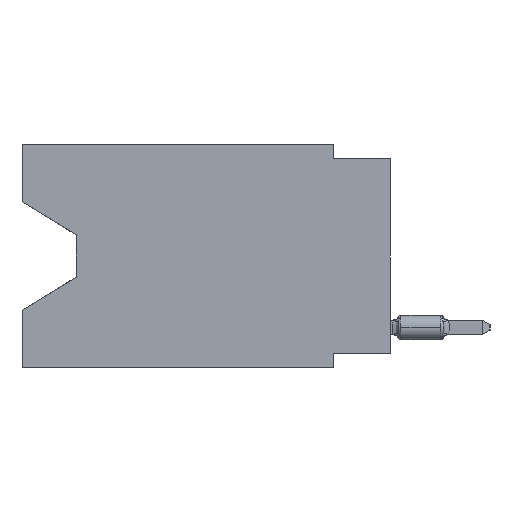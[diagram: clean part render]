
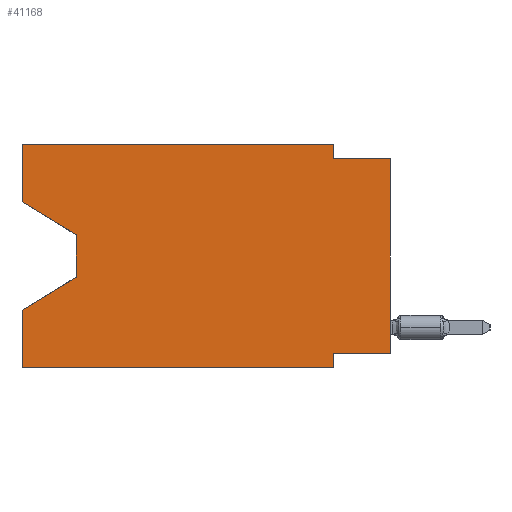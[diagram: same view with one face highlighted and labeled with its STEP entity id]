
A CAD part, left-side view. The second image highlights one B-rep face of the part: STEP entity #41168.
In plain terms, the highlighted planar face has unit normal (-1, 0, 0).
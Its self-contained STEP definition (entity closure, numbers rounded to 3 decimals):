
#561 = EDGE_CURVE ( 'NONE', #10498, #40357, #6008, .T. ) ;
#677 = DIRECTION ( 'NONE',  ( 0., -0.855, -0.519 ) ) ;
#1276 = CARTESIAN_POINT ( 'NONE',  ( 0., 0., 0. ) ) ;
#1778 = CARTESIAN_POINT ( 'NONE',  ( 0., 13.97, -4.013 ) ) ;
#1964 = CARTESIAN_POINT ( 'NONE',  ( 0., 0., -9.271 ) ) ;
#2694 = VERTEX_POINT ( 'NONE', #9017 ) ;
#3584 = VECTOR ( 'NONE', #27656, 1000. ) ;
#3711 = ORIENTED_EDGE ( 'NONE', *, *, #38095, .F. ) ;
#3873 = ORIENTED_EDGE ( 'NONE', *, *, #47036, .F. ) ;
#3886 = CARTESIAN_POINT ( 'NONE',  ( 0., 13.97, -5.893 ) ) ;
#4195 = LINE ( 'NONE', #28365, #49214 ) ;
#4669 = EDGE_CURVE ( 'NONE', #34271, #47103, #37674, .T. ) ;
#5193 = FACE_OUTER_BOUND ( 'NONE', #19505, .T. ) ;
#5781 = CARTESIAN_POINT ( 'NONE',  ( 0., 16.383, 0. ) ) ;
#6008 = LINE ( 'NONE', #1778, #26096 ) ;
#6830 = VECTOR ( 'NONE', #31070, 1000. ) ;
#7678 = VECTOR ( 'NONE', #21183, 1000. ) ;
#8118 = DIRECTION ( 'NONE',  ( 0., 0.855, -0.519 ) ) ;
#8648 = ORIENTED_EDGE ( 'NONE', *, *, #561, .T. ) ;
#9017 = CARTESIAN_POINT ( 'NONE',  ( 0., 16.383, -9.906 ) ) ;
#9403 = CARTESIAN_POINT ( 'NONE',  ( 0., 16.383, 0. ) ) ;
#10498 = VERTEX_POINT ( 'NONE', #44036 ) ;
#11215 = DIRECTION ( 'NONE',  ( 0., 0., -1. ) ) ;
#11441 = CARTESIAN_POINT ( 'NONE',  ( 0., 16.383, 0. ) ) ;
#11472 = CARTESIAN_POINT ( 'NONE',  ( 0., 2.54, 0. ) ) ;
#11843 = CARTESIAN_POINT ( 'NONE',  ( 0., 16.383, -7.36 ) ) ;
#12402 = CARTESIAN_POINT ( 'NONE',  ( 0., 2.54, -9.271 ) ) ;
#14045 = CARTESIAN_POINT ( 'NONE',  ( 0., 16.383, -9.906 ) ) ;
#14407 = ORIENTED_EDGE ( 'NONE', *, *, #51488, .F. ) ;
#16347 = ORIENTED_EDGE ( 'NONE', *, *, #43028, .T. ) ;
#16636 = ORIENTED_EDGE ( 'NONE', *, *, #39897, .T. ) ;
#16819 = DIRECTION ( 'NONE',  ( 0., 1., 0. ) ) ;
#17149 = VERTEX_POINT ( 'NONE', #5781 ) ;
#17970 = VERTEX_POINT ( 'NONE', #35921 ) ;
#18001 = CARTESIAN_POINT ( 'NONE',  ( 0., 0., -0.635 ) ) ;
#18196 = DIRECTION ( 'NONE',  ( 1., 0., 0. ) ) ;
#19505 = EDGE_LOOP ( 'NONE', ( #16636, #8648, #44319, #31109, #16347, #34948, #3711, #27749, #3873, #35640, #29774, #14407 ) ) ;
#20395 = DIRECTION ( 'NONE',  ( 0., 0., 1. ) ) ;
#20474 = VERTEX_POINT ( 'NONE', #37062 ) ;
#21049 = LINE ( 'NONE', #3886, #47993 ) ;
#21183 = DIRECTION ( 'NONE',  ( 0., -1., 0. ) ) ;
#21549 = EDGE_CURVE ( 'NONE', #26577, #20474, #44074, .T. ) ;
#22024 = LINE ( 'NONE', #14045, #49543 ) ;
#24725 = CARTESIAN_POINT ( 'NONE',  ( 0., 13.97, -5.893 ) ) ;
#25175 = CARTESIAN_POINT ( 'NONE',  ( 0., 0., -0.635 ) ) ;
#25344 = EDGE_CURVE ( 'NONE', #2694, #36267, #4195, .T. ) ;
#26096 = VECTOR ( 'NONE', #50118, 1000. ) ;
#26577 = VERTEX_POINT ( 'NONE', #12402 ) ;
#27268 = CARTESIAN_POINT ( 'NONE',  ( 0., 2.54, -0.635 ) ) ;
#27656 = DIRECTION ( 'NONE',  ( 0., 0., 1. ) ) ;
#27749 = ORIENTED_EDGE ( 'NONE', *, *, #4669, .T. ) ;
#28365 = CARTESIAN_POINT ( 'NONE',  ( 0., 16.383, 0. ) ) ;
#28625 = LINE ( 'NONE', #25175, #7678 ) ;
#29295 = LINE ( 'NONE', #45507, #32343 ) ;
#29618 = DIRECTION ( 'NONE',  ( 0., 0., -1. ) ) ;
#29774 = ORIENTED_EDGE ( 'NONE', *, *, #46326, .F. ) ;
#31070 = DIRECTION ( 'NONE',  ( 0., 0., -1. ) ) ;
#31109 = ORIENTED_EDGE ( 'NONE', *, *, #25344, .F. ) ;
#32343 = VECTOR ( 'NONE', #16819, 1000. ) ;
#34110 = LINE ( 'NONE', #9403, #47356 ) ;
#34271 = VERTEX_POINT ( 'NONE', #1964 ) ;
#34670 = CARTESIAN_POINT ( 'NONE',  ( 0., 16.383, 0. ) ) ;
#34948 = ORIENTED_EDGE ( 'NONE', *, *, #21549, .F. ) ;
#35640 = ORIENTED_EDGE ( 'NONE', *, *, #38329, .F. ) ;
#35921 = CARTESIAN_POINT ( 'NONE',  ( 0., 2.54, 0. ) ) ;
#36267 = VERTEX_POINT ( 'NONE', #11843 ) ;
#37062 = CARTESIAN_POINT ( 'NONE',  ( 0., 2.54, -9.906 ) ) ;
#37508 = CARTESIAN_POINT ( 'NONE',  ( 0., 16.383, -2.546 ) ) ;
#37674 = LINE ( 'NONE', #1276, #44317 ) ;
#38095 = EDGE_CURVE ( 'NONE', #34271, #26577, #29295, .T. ) ;
#38329 = EDGE_CURVE ( 'NONE', #17970, #52236, #47886, .T. ) ;
#39897 = EDGE_CURVE ( 'NONE', #43920, #10498, #44270, .T. ) ;
#40280 = CARTESIAN_POINT ( 'NONE',  ( 0., 16.383, -2.546 ) ) ;
#40357 = VERTEX_POINT ( 'NONE', #24725 ) ;
#41168 = ADVANCED_FACE ( 'NONE', ( #5193 ), #41849, .F. ) ;
#41822 = DIRECTION ( 'NONE',  ( 0., -1., 0. ) ) ;
#41849 = PLANE ( 'NONE',  #47034 ) ;
#43028 = EDGE_CURVE ( 'NONE', #2694, #20474, #22024, .T. ) ;
#43356 = LINE ( 'NONE', #11441, #3584 ) ;
#43920 = VERTEX_POINT ( 'NONE', #37508 ) ;
#44036 = CARTESIAN_POINT ( 'NONE',  ( 0., 13.97, -4.013 ) ) ;
#44074 = LINE ( 'NONE', #51516, #6830 ) ;
#44270 = LINE ( 'NONE', #40280, #48638 ) ;
#44317 = VECTOR ( 'NONE', #49880, 1000. ) ;
#44319 = ORIENTED_EDGE ( 'NONE', *, *, #52370, .T. ) ;
#45507 = CARTESIAN_POINT ( 'NONE',  ( 0., 0., -9.271 ) ) ;
#46326 = EDGE_CURVE ( 'NONE', #17149, #17970, #34110, .T. ) ;
#46473 = DIRECTION ( 'NONE',  ( 0., -1., 0. ) ) ;
#47034 = AXIS2_PLACEMENT_3D ( 'NONE', #34670, #18196, #29618 ) ;
#47036 = EDGE_CURVE ( 'NONE', #52236, #47103, #28625, .T. ) ;
#47103 = VERTEX_POINT ( 'NONE', #18001 ) ;
#47356 = VECTOR ( 'NONE', #41822, 1000. ) ;
#47886 = LINE ( 'NONE', #11472, #50203 ) ;
#47993 = VECTOR ( 'NONE', #8118, 1000. ) ;
#48638 = VECTOR ( 'NONE', #677, 1000. ) ;
#49214 = VECTOR ( 'NONE', #20395, 1000. ) ;
#49543 = VECTOR ( 'NONE', #46473, 1000. ) ;
#49880 = DIRECTION ( 'NONE',  ( 0., 0., 1. ) ) ;
#50118 = DIRECTION ( 'NONE',  ( 0., 0., -1. ) ) ;
#50203 = VECTOR ( 'NONE', #11215, 1000. ) ;
#51488 = EDGE_CURVE ( 'NONE', #43920, #17149, #43356, .T. ) ;
#51516 = CARTESIAN_POINT ( 'NONE',  ( 0., 2.54, -9.906 ) ) ;
#52236 = VERTEX_POINT ( 'NONE', #27268 ) ;
#52370 = EDGE_CURVE ( 'NONE', #40357, #36267, #21049, .T. ) ;
